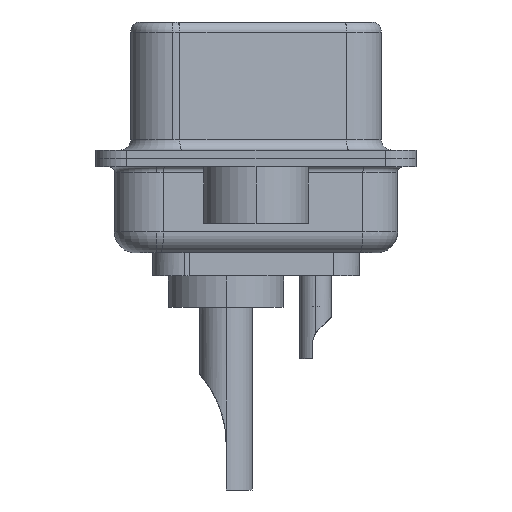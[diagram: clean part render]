
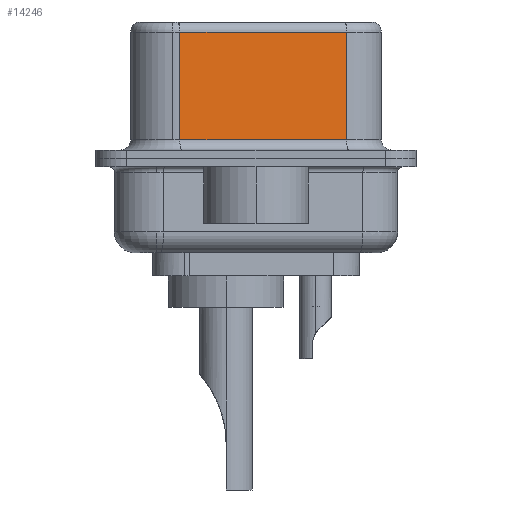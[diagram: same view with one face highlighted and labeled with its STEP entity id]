
A CAD part, left-side view. The second image highlights one B-rep face of the part: STEP entity #14246.
In plain terms, the highlighted planar face has unit normal (-0.985, -0.174, 0).
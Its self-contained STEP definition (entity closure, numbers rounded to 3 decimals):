
#69 = FACE_OUTER_BOUND ( 'NONE', #11533, .T. ) ;
#833 = LINE ( 'NONE', #23637, #10196 ) ;
#838 = CARTESIAN_POINT ( 'NONE',  ( 3.73, 3.628, 6.02 ) ) ;
#1006 = CARTESIAN_POINT ( 'NONE',  ( 5.132, -4.322, 6.52 ) ) ;
#1085 = DIRECTION ( 'NONE',  ( -0.174, 0.985, 0. ) ) ;
#1183 = DIRECTION ( 'NONE',  ( 0., 0., -1. ) ) ;
#1810 = CARTESIAN_POINT ( 'NONE',  ( 5.132, -4.322, 6.02 ) ) ;
#2520 = VERTEX_POINT ( 'NONE', #1810 ) ;
#3808 = CARTESIAN_POINT ( 'NONE',  ( 3.73, 3.628, 0.9 ) ) ;
#4440 = VECTOR ( 'NONE', #23070, 1000. ) ;
#5137 = EDGE_CURVE ( 'NONE', #2520, #16457, #833, .T. ) ;
#8092 = CARTESIAN_POINT ( 'NONE',  ( 5.132, -4.322, 0.9 ) ) ;
#8525 = PLANE ( 'NONE',  #19882 ) ;
#9230 = EDGE_CURVE ( 'NONE', #13875, #23584, #19392, .T. ) ;
#9854 = ORIENTED_EDGE ( 'NONE', *, *, #22249, .F. ) ;
#10196 = VECTOR ( 'NONE', #22816, 1000. ) ;
#10228 = LINE ( 'NONE', #16169, #14629 ) ;
#11533 = EDGE_LOOP ( 'NONE', ( #9854, #15355, #14459, #18683 ) ) ;
#12065 = DIRECTION ( 'NONE',  ( 0., 0., -1. ) ) ;
#12311 = DIRECTION ( 'NONE',  ( 0.985, 0.174, 0. ) ) ;
#13875 = VERTEX_POINT ( 'NONE', #3808 ) ;
#13950 = CARTESIAN_POINT ( 'NONE',  ( 3.73, 3.628, 6.52 ) ) ;
#14246 = ADVANCED_FACE ( 'NONE', ( #69 ), #8525, .F. ) ;
#14437 = LINE ( 'NONE', #13950, #18839 ) ;
#14459 = ORIENTED_EDGE ( 'NONE', *, *, #18682, .T. ) ;
#14629 = VECTOR ( 'NONE', #1183, 1000. ) ;
#15355 = ORIENTED_EDGE ( 'NONE', *, *, #5137, .T. ) ;
#16169 = CARTESIAN_POINT ( 'NONE',  ( 5.132, -4.322, 6.52 ) ) ;
#16450 = CARTESIAN_POINT ( 'NONE',  ( 5.132, -4.322, 0.9 ) ) ;
#16457 = VERTEX_POINT ( 'NONE', #838 ) ;
#18682 = EDGE_CURVE ( 'NONE', #16457, #13875, #14437, .T. ) ;
#18683 = ORIENTED_EDGE ( 'NONE', *, *, #9230, .T. ) ;
#18839 = VECTOR ( 'NONE', #12065, 1000. ) ;
#19392 = LINE ( 'NONE', #8092, #4440 ) ;
#19882 = AXIS2_PLACEMENT_3D ( 'NONE', #1006, #12311, #1085 ) ;
#22249 = EDGE_CURVE ( 'NONE', #2520, #23584, #10228, .T. ) ;
#22816 = DIRECTION ( 'NONE',  ( -0.174, 0.985, 0. ) ) ;
#23070 = DIRECTION ( 'NONE',  ( 0.174, -0.985, 0. ) ) ;
#23584 = VERTEX_POINT ( 'NONE', #16450 ) ;
#23637 = CARTESIAN_POINT ( 'NONE',  ( 5.132, -4.322, 6.02 ) ) ;
